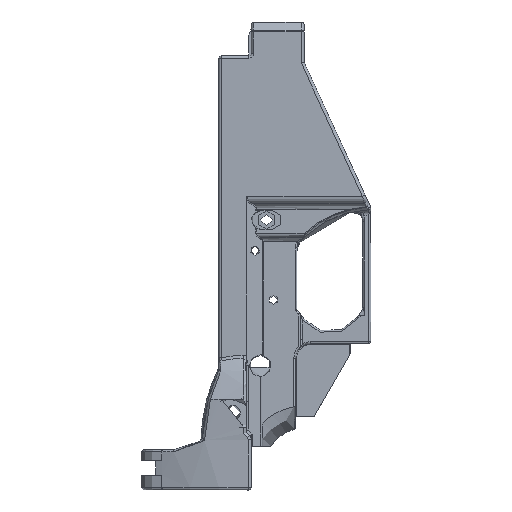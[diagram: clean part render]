
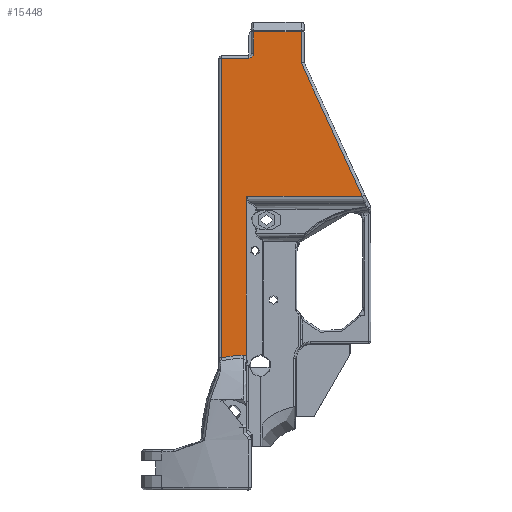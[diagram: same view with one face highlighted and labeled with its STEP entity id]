
A CAD part, left-side view. The second image highlights one B-rep face of the part: STEP entity #15448.
In plain terms, the highlighted planar face has unit normal (-1, 0, 0).
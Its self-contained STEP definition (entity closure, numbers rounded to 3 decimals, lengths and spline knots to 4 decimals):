
#219=ELLIPSE('',#16831,1.9201,1.636);
#396=PLANE('',#16829);
#1334=FACE_OUTER_BOUND('',#2282,.T.);
#2282=EDGE_LOOP('',(#12417,#12418,#12419,#12420,#12421,#12422,#12423,#12424,
#12425,#12426,#12427,#12428));
#3233=B_SPLINE_CURVE_WITH_KNOTS('',3,(#43339,#43340,#43341,#43342),
 .UNSPECIFIED.,.F.,.F.,(4,4),(-0.1434,0.),
 .UNSPECIFIED.);
#3234=B_SPLINE_CURVE_WITH_KNOTS('',3,(#43346,#43347,#43348,#43349,#43350,
#43351,#43352,#43353,#43354,#43355,#43356,#43357),.UNSPECIFIED.,.F.,.F.,
(4,2,2,2,2,4),(-0.117,-0.1147,-0.0798,
-0.057,-0.0072,0.),.UNSPECIFIED.);
#3857=CIRCLE('',#16830,0.08);
#4492=LINE('',#25868,#5261);
#4494=LINE('',#25899,#5263);
#4674=LINE('',#43291,#5443);
#4678=LINE('',#43329,#5447);
#4679=LINE('',#43333,#5448);
#4680=LINE('',#43335,#5449);
#4681=LINE('',#43344,#5450);
#4682=LINE('',#43358,#5451);
#5261=VECTOR('',#19021,0.3937);
#5263=VECTOR('',#19033,0.3937);
#5443=VECTOR('',#19863,0.3937);
#5447=VECTOR('',#19885,0.3937);
#5448=VECTOR('',#19888,0.3937);
#5449=VECTOR('',#19889,0.3937);
#5450=VECTOR('',#19892,1.6985);
#5451=VECTOR('',#19893,0.1181);
#6263=VERTEX_POINT('',#25865);
#6264=VERTEX_POINT('',#25867);
#6268=VERTEX_POINT('',#25897);
#6772=VERTEX_POINT('',#43289);
#6777=VERTEX_POINT('',#43328);
#6778=VERTEX_POINT('',#43330);
#6779=VERTEX_POINT('',#43332);
#6780=VERTEX_POINT('',#43334);
#6781=VERTEX_POINT('',#43336);
#6782=VERTEX_POINT('',#43338);
#6783=VERTEX_POINT('',#43343);
#6784=VERTEX_POINT('',#43345);
#8040=EDGE_CURVE('',#6263,#6264,#4492,.T.);
#8047=EDGE_CURVE('',#6268,#6263,#4494,.T.);
#8783=EDGE_CURVE('',#6772,#6268,#4674,.T.);
#8792=EDGE_CURVE('',#6777,#6772,#4678,.T.);
#8793=EDGE_CURVE('',#6778,#6777,#3857,.T.);
#8794=EDGE_CURVE('',#6779,#6778,#4679,.T.);
#8795=EDGE_CURVE('',#6780,#6779,#4680,.T.);
#8796=EDGE_CURVE('',#6781,#6780,#219,.T.);
#8797=EDGE_CURVE('',#6782,#6781,#3233,.T.);
#8798=EDGE_CURVE('',#6783,#6782,#4681,.T.);
#8799=EDGE_CURVE('',#6784,#6783,#3234,.T.);
#8800=EDGE_CURVE('',#6264,#6784,#4682,.T.);
#12417=ORIENTED_EDGE('',*,*,#8040,.F.);
#12418=ORIENTED_EDGE('',*,*,#8047,.F.);
#12419=ORIENTED_EDGE('',*,*,#8783,.F.);
#12420=ORIENTED_EDGE('',*,*,#8792,.F.);
#12421=ORIENTED_EDGE('',*,*,#8793,.F.);
#12422=ORIENTED_EDGE('',*,*,#8794,.F.);
#12423=ORIENTED_EDGE('',*,*,#8795,.F.);
#12424=ORIENTED_EDGE('',*,*,#8796,.F.);
#12425=ORIENTED_EDGE('',*,*,#8797,.F.);
#12426=ORIENTED_EDGE('',*,*,#8798,.F.);
#12427=ORIENTED_EDGE('',*,*,#8799,.F.);
#12428=ORIENTED_EDGE('',*,*,#8800,.F.);
#15448=ADVANCED_FACE('',(#1334),#396,.F.);
#16829=AXIS2_PLACEMENT_3D('',#43327,#19883,#19884);
#16830=AXIS2_PLACEMENT_3D('',#43331,#19886,#19887);
#16831=AXIS2_PLACEMENT_3D('',#43337,#19890,#19891);
#19021=DIRECTION('',(0.,-0.417,-0.909));
#19033=DIRECTION('',(0.,0.,-1.));
#19863=DIRECTION('',(0.,-1.,0.));
#19883=DIRECTION('center_axis',(1.,0.,0.));
#19884=DIRECTION('ref_axis',(0.,0.,
-1.));
#19885=DIRECTION('',(0.,0.,1.));
#19886=DIRECTION('center_axis',(-1.,0.,0.));
#19887=DIRECTION('ref_axis',(0.,-0.707,-0.707));
#19888=DIRECTION('',(0.,-1.,0.));
#19889=DIRECTION('',(0.,0.,1.));
#19890=DIRECTION('center_axis',(-1.,0.,0.));
#19891=DIRECTION('ref_axis',(0.,-0.984,-0.179));
#19892=DIRECTION('',(0.,0.,-1.));
#19893=DIRECTION('',(0.,1.,0.));
#25865=CARTESIAN_POINT('',(-0.731,-0.0727,2.8507));
#25867=CARTESIAN_POINT('',(-0.731,-1.118,0.5717));
#25868=CARTESIAN_POINT('',(-0.731,-1.4648,-0.1846));
#25897=CARTESIAN_POINT('',(-0.731,-0.0728,3.3816));
#25899=CARTESIAN_POINT('',(-0.731,-0.0727,-0.2092));
#43289=CARTESIAN_POINT('',(-0.731,0.7372,3.3816));
#43291=CARTESIAN_POINT('',(-0.731,0.7121,3.3816));
#43327=CARTESIAN_POINT('Origin',(-0.731,0.68,-3.6849));
#43328=CARTESIAN_POINT('',(-0.731,0.7373,3.0095));
#43329=CARTESIAN_POINT('',(-0.731,0.7373,-0.0118));
#43330=CARTESIAN_POINT('',(-0.731,0.8173,2.9295));
#43331=CARTESIAN_POINT('Origin',(-0.731,0.8173,3.0095));
#43332=CARTESIAN_POINT('',(-0.731,1.2902,2.9295));
#43333=CARTESIAN_POINT('',(-0.731,0.7441,2.9295));
#43334=CARTESIAN_POINT('',(-0.731,1.2902,-2.1813));
#43335=CARTESIAN_POINT('',(-0.731,1.2902,-3.1756));
#43336=CARTESIAN_POINT('',(-0.731,0.9158,-2.1342));
#43337=CARTESIAN_POINT('Origin',(-0.731,0.7244,-3.7785));
#43338=CARTESIAN_POINT('',(-0.731,0.8628,-2.151));
#43339=CARTESIAN_POINT('Ctrl Pts',(-0.731,0.8629,
-2.151));
#43340=CARTESIAN_POINT('Ctrl Pts',(-0.731,0.8784,
-2.1404));
#43341=CARTESIAN_POINT('Ctrl Pts',(-0.731,0.8969,
-2.1335));
#43342=CARTESIAN_POINT('Ctrl Pts',(-0.731,0.9158,
-2.1342));
#43343=CARTESIAN_POINT('',(-0.731,0.8628,0.5319));
#43344=CARTESIAN_POINT('',(-0.731,0.8628,-2.5001));
#43345=CARTESIAN_POINT('',(-0.731,0.8546,0.5717));
#43346=CARTESIAN_POINT('Ctrl Pts',(-0.731,0.8546,
0.5717));
#43347=CARTESIAN_POINT('Ctrl Pts',(-0.731,0.8546,
0.5716));
#43348=CARTESIAN_POINT('Ctrl Pts',(-0.731,0.8546,
0.5716));
#43349=CARTESIAN_POINT('Ctrl Pts',(-0.731,0.855,
0.5706));
#43350=CARTESIAN_POINT('Ctrl Pts',(-0.731,0.8564,
0.5674));
#43351=CARTESIAN_POINT('Ctrl Pts',(-0.731,0.8587,
0.5601));
#43352=CARTESIAN_POINT('Ctrl Pts',(-0.731,0.8595,
0.5572));
#43353=CARTESIAN_POINT('Ctrl Pts',(-0.731,0.8617,
0.5478));
#43354=CARTESIAN_POINT('Ctrl Pts',(-0.731,0.8626,
0.5413));
#43355=CARTESIAN_POINT('Ctrl Pts',(-0.731,0.8628,
0.5338));
#43356=CARTESIAN_POINT('Ctrl Pts',(-0.731,0.8628,
0.5329));
#43357=CARTESIAN_POINT('Ctrl Pts',(-0.731,0.8628,
0.5319));
#43358=CARTESIAN_POINT('',(-0.731,1.0895,0.5717));
